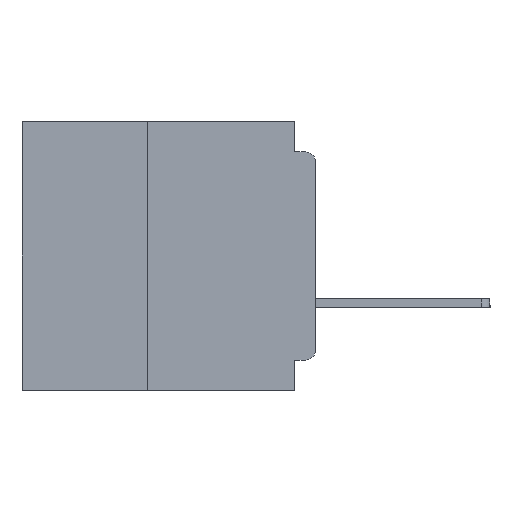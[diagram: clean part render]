
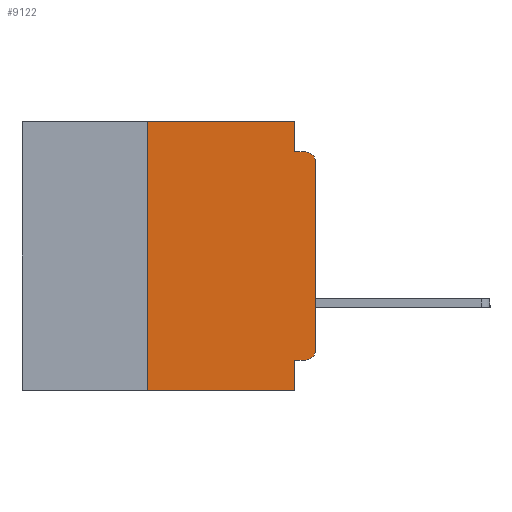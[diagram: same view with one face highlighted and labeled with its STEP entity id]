
A CAD part, left-side view. The second image highlights one B-rep face of the part: STEP entity #9122.
In plain terms, the highlighted planar face has unit normal (-1, 0, 0).
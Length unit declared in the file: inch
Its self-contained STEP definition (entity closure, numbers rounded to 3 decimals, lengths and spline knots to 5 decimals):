
#725 = ORIENTED_EDGE ( 'NONE', *, *, #1320, .F. ) ;
#1320 = EDGE_CURVE ( 'NONE', #10635, #44733, #35640, .T. ) ;
#1716 = EDGE_CURVE ( 'NONE', #32276, #7376, #17181, .T. ) ;
#1815 = DIRECTION ( 'NONE',  ( 0., 0., -1. ) ) ;
#2991 = EDGE_CURVE ( 'NONE', #12829, #44733, #7858, .T. ) ;
#4351 = VECTOR ( 'NONE', #39955, 39.37008 ) ;
#5042 = LINE ( 'NONE', #25295, #45376 ) ;
#5342 = DIRECTION ( 'NONE',  ( 0., 0., 1. ) ) ;
#6243 = DIRECTION ( 'NONE',  ( 0., 0., 1. ) ) ;
#6494 = LINE ( 'NONE', #40550, #15697 ) ;
#7376 = VERTEX_POINT ( 'NONE', #49941 ) ;
#7429 = CARTESIAN_POINT ( 'NONE',  ( 0., 0., 0. ) ) ;
#7457 = CARTESIAN_POINT ( 'NONE',  ( 0., 0.015, -0.045 ) ) ;
#7462 = VERTEX_POINT ( 'NONE', #7719 ) ;
#7719 = CARTESIAN_POINT ( 'NONE',  ( 0., 0.031, -0.045 ) ) ;
#7858 = LINE ( 'NONE', #37787, #48065 ) ;
#8111 = EDGE_CURVE ( 'NONE', #36107, #36912, #29611, .T. ) ;
#8547 = CIRCLE ( 'NONE', #45294, 0.015 ) ;
#9122 = ADVANCED_FACE ( 'NONE', ( #36233 ), #34663, .F. ) ;
#10293 = VERTEX_POINT ( 'NONE', #7457 ) ;
#10635 = VERTEX_POINT ( 'NONE', #44810 ) ;
#11172 = VECTOR ( 'NONE', #11897, 39.37008 ) ;
#11897 = DIRECTION ( 'NONE',  ( 0., -1., 0. ) ) ;
#12055 = CARTESIAN_POINT ( 'NONE',  ( 0., 0.015, -0.06 ) ) ;
#12829 = VERTEX_POINT ( 'NONE', #16112 ) ;
#12877 = DIRECTION ( 'NONE',  ( -1., 0., 0. ) ) ;
#12891 = CIRCLE ( 'NONE', #42624, 0.015 ) ;
#13209 = CARTESIAN_POINT ( 'NONE',  ( 0., 0.25, -0.4 ) ) ;
#14174 = EDGE_CURVE ( 'NONE', #7462, #10293, #6494, .T. ) ;
#14902 = CARTESIAN_POINT ( 'NONE',  ( 0., 0.015, -0.355 ) ) ;
#15118 = DIRECTION ( 'NONE',  ( 1., 0., 0. ) ) ;
#15289 = ORIENTED_EDGE ( 'NONE', *, *, #34536, .F. ) ;
#15359 = VECTOR ( 'NONE', #19821, 39.37008 ) ;
#15697 = VECTOR ( 'NONE', #44373, 39.37008 ) ;
#15718 = VERTEX_POINT ( 'NONE', #14902 ) ;
#16033 = DIRECTION ( 'NONE',  ( 0., 0., -1. ) ) ;
#16112 = CARTESIAN_POINT ( 'NONE',  ( 0., 0.25, -0.4 ) ) ;
#17181 = LINE ( 'NONE', #7429, #36833 ) ;
#18720 = EDGE_CURVE ( 'NONE', #12829, #36107, #36124, .T. ) ;
#19821 = DIRECTION ( 'NONE',  ( 0., 1., 0. ) ) ;
#21676 = EDGE_CURVE ( 'NONE', #7376, #10293, #12891, .T. ) ;
#23226 = VECTOR ( 'NONE', #5342, 39.37008 ) ;
#24549 = LINE ( 'NONE', #43222, #15359 ) ;
#25295 = CARTESIAN_POINT ( 'NONE',  ( 0., 0.031, 0. ) ) ;
#25712 = ORIENTED_EDGE ( 'NONE', *, *, #48655, .T. ) ;
#25925 = CARTESIAN_POINT ( 'NONE',  ( 0., 0., -0.34 ) ) ;
#26977 = CARTESIAN_POINT ( 'NONE',  ( 0., 0.031, 0. ) ) ;
#28253 = ORIENTED_EDGE ( 'NONE', *, *, #21676, .T. ) ;
#29611 = LINE ( 'NONE', #35425, #11172 ) ;
#30535 = CARTESIAN_POINT ( 'NONE',  ( 0., 0.437, 0. ) ) ;
#30724 = ORIENTED_EDGE ( 'NONE', *, *, #1716, .T. ) ;
#31213 = ORIENTED_EDGE ( 'NONE', *, *, #18720, .F. ) ;
#31296 = EDGE_LOOP ( 'NONE', ( #30724, #28253, #45825, #15289, #34921, #31213, #46907, #725, #46898, #25712 ) ) ;
#32184 = CARTESIAN_POINT ( 'NONE',  ( 0., 0.031, -0.4 ) ) ;
#32276 = VERTEX_POINT ( 'NONE', #25925 ) ;
#33751 = CARTESIAN_POINT ( 'NONE',  ( 0., 0.25, 0. ) ) ;
#34536 = EDGE_CURVE ( 'NONE', #36912, #7462, #5042, .T. ) ;
#34663 = PLANE ( 'NONE',  #46901 ) ;
#34921 = ORIENTED_EDGE ( 'NONE', *, *, #8111, .F. ) ;
#35425 = CARTESIAN_POINT ( 'NONE',  ( 0., 0.437, 0. ) ) ;
#35640 = LINE ( 'NONE', #40337, #4351 ) ;
#36107 = VERTEX_POINT ( 'NONE', #33751 ) ;
#36124 = LINE ( 'NONE', #13209, #23226 ) ;
#36233 = FACE_OUTER_BOUND ( 'NONE', #31296, .T. ) ;
#36392 = CARTESIAN_POINT ( 'NONE',  ( 0., 0.015, -0.34 ) ) ;
#36833 = VECTOR ( 'NONE', #6243, 39.37008 ) ;
#36912 = VERTEX_POINT ( 'NONE', #26977 ) ;
#37193 = DIRECTION ( 'NONE',  ( 0., -1., 0. ) ) ;
#37787 = CARTESIAN_POINT ( 'NONE',  ( 0., 0.437, -0.4 ) ) ;
#39091 = EDGE_CURVE ( 'NONE', #15718, #10635, #24549, .T. ) ;
#39520 = DIRECTION ( 'NONE',  ( -1., 0., 0. ) ) ;
#39955 = DIRECTION ( 'NONE',  ( 0., 0., -1. ) ) ;
#40312 = DIRECTION ( 'NONE',  ( 0., 0., -1. ) ) ;
#40337 = CARTESIAN_POINT ( 'NONE',  ( 0., 0.031, -0.4 ) ) ;
#40550 = CARTESIAN_POINT ( 'NONE',  ( 0., 0., -0.045 ) ) ;
#42466 = DIRECTION ( 'NONE',  ( 0., 0., -1. ) ) ;
#42624 = AXIS2_PLACEMENT_3D ( 'NONE', #12055, #39520, #16033 ) ;
#43222 = CARTESIAN_POINT ( 'NONE',  ( 0., 0., -0.355 ) ) ;
#44373 = DIRECTION ( 'NONE',  ( 0., -1., 0. ) ) ;
#44733 = VERTEX_POINT ( 'NONE', #32184 ) ;
#44810 = CARTESIAN_POINT ( 'NONE',  ( 0., 0.031, -0.355 ) ) ;
#45294 = AXIS2_PLACEMENT_3D ( 'NONE', #36392, #12877, #40312 ) ;
#45376 = VECTOR ( 'NONE', #1815, 39.37008 ) ;
#45825 = ORIENTED_EDGE ( 'NONE', *, *, #14174, .F. ) ;
#46898 = ORIENTED_EDGE ( 'NONE', *, *, #39091, .F. ) ;
#46901 = AXIS2_PLACEMENT_3D ( 'NONE', #30535, #15118, #42466 ) ;
#46907 = ORIENTED_EDGE ( 'NONE', *, *, #2991, .T. ) ;
#48065 = VECTOR ( 'NONE', #37193, 39.37008 ) ;
#48655 = EDGE_CURVE ( 'NONE', #15718, #32276, #8547, .T. ) ;
#49941 = CARTESIAN_POINT ( 'NONE',  ( 0., 0., -0.06 ) ) ;
